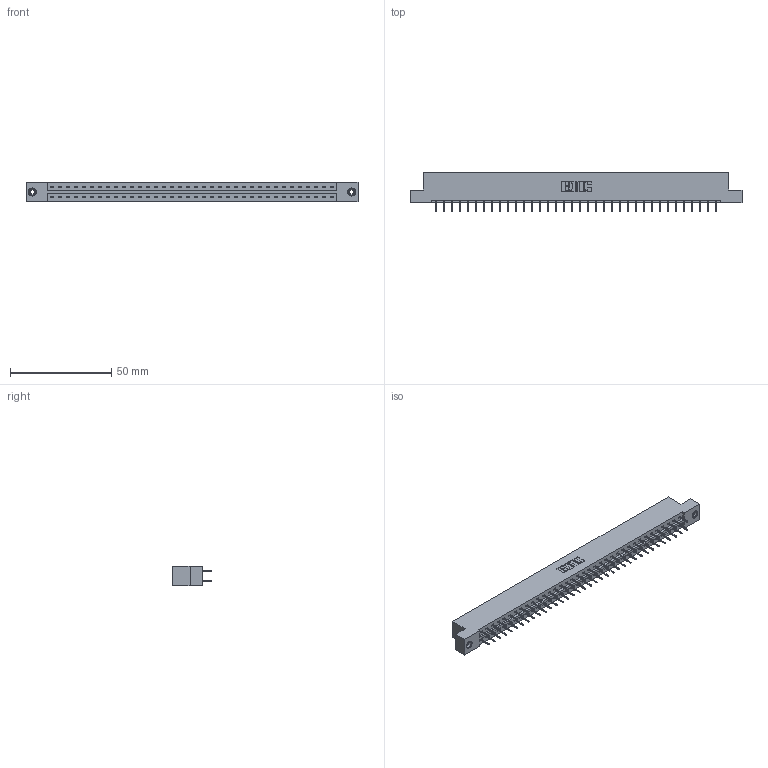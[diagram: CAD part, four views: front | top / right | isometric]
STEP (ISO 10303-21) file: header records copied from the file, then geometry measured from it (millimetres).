
FILE_DESCRIPTION (( 'STEP AP203' ), '1' );
FILE_NAME ('833-072-524-208.STEP', '2020-06-05T14:04:16', ( '' ), ( '' ), 'SwSTEP 2.0', 'SolidWorks 2020', '' );
FILE_SCHEMA (( 'CONFIG_CONTROL_DESIGN' ));
Length unit declared in the file: inch
Products named in the file (4): 833 Part_Flush - .156 Dia - TI; 345-292-001_345-293-124; 833-072-524-208; 345-250-001_345-250-003-102
Assembly tree (75 placements, depth 2):
  833-072-524-208
    833 Part_Flush - .156 Dia - TI
    345-292-001_345-293-124  x72
    345-250-001_345-250-003-102  x2
Bounding box: 164.19 x 19.69 x 9.4 mm (x, y, z)
Volume: 16590.8 mm3; surface area: 19244.7 mm2
Topology: 75 solids, 75 shells, 4206 faces, 11895 edges, 7634 vertices
Faces by surface type: plane 3126, cylinder 1064, cone 12, torus 4
Entity records: 25196 total; most frequent: CARTESIAN_POINT 4165, ORIENTED_EDGE 4094, DIRECTION 3601, EDGE_CURVE 2047, LINE 1903, VECTOR 1903, VERTEX_POINT 1356, AXIS2_PLACEMENT_3D 849
